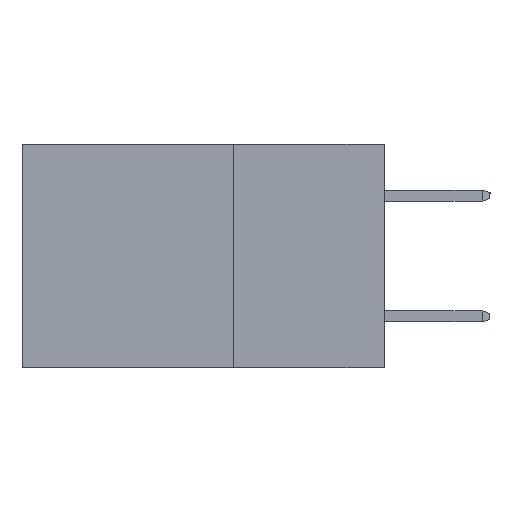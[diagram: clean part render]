
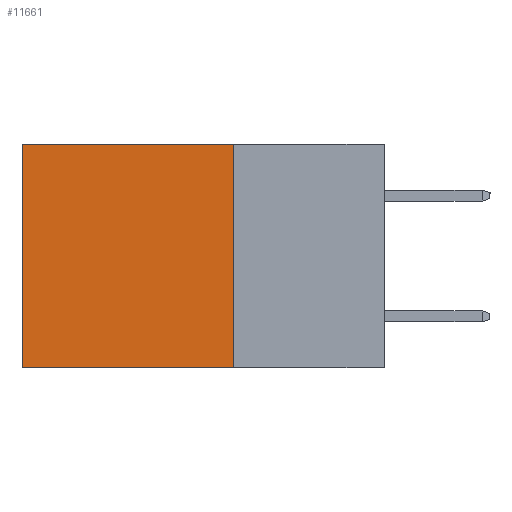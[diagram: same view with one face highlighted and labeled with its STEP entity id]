
A CAD part, left-side view. The second image highlights one B-rep face of the part: STEP entity #11661.
In plain terms, the highlighted planar face has unit normal (-1, 0, 0).
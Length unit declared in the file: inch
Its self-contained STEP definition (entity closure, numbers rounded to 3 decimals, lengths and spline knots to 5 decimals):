
#62 = LINE ( 'NONE', #4975, #13554 ) ;
#222 = EDGE_CURVE ( 'NONE', #4156, #1434, #7986, .T. ) ;
#230 = VERTEX_POINT ( 'NONE', #12919 ) ;
#1212 = CARTESIAN_POINT ( 'NONE',  ( 0.2615, 0.25, 0. ) ) ;
#1434 = VERTEX_POINT ( 'NONE', #3114 ) ;
#1591 = EDGE_CURVE ( 'NONE', #6395, #4156, #9909, .T. ) ;
#1595 = DIRECTION ( 'NONE',  ( 0., 0., -1. ) ) ;
#2038 = VECTOR ( 'NONE', #6768, 39.37008 ) ;
#2165 = PLANE ( 'NONE',  #11972 ) ;
#3040 = CARTESIAN_POINT ( 'NONE',  ( 0.2615, 0.6, -0.37 ) ) ;
#3114 = CARTESIAN_POINT ( 'NONE',  ( 0.2615, 0.6, -0.37 ) ) ;
#4156 = VERTEX_POINT ( 'NONE', #8247 ) ;
#4810 = CARTESIAN_POINT ( 'NONE',  ( 0.2615, 0.25, 0. ) ) ;
#4944 = ORIENTED_EDGE ( 'NONE', *, *, #222, .T. ) ;
#4975 = CARTESIAN_POINT ( 'NONE',  ( 0.2615, 0.25, -0.37 ) ) ;
#5056 = DIRECTION ( 'NONE',  ( 0., 1., 0. ) ) ;
#6395 = VERTEX_POINT ( 'NONE', #1212 ) ;
#6768 = DIRECTION ( 'NONE',  ( 0., 0., -1. ) ) ;
#7550 = ORIENTED_EDGE ( 'NONE', *, *, #1591, .T. ) ;
#7751 = LINE ( 'NONE', #9049, #14523 ) ;
#7986 = LINE ( 'NONE', #3040, #2038 ) ;
#8247 = CARTESIAN_POINT ( 'NONE',  ( 0.2615, 0.6, 0. ) ) ;
#9049 = CARTESIAN_POINT ( 'NONE',  ( 0.2615, 0.25, -0.37 ) ) ;
#9702 = CARTESIAN_POINT ( 'NONE',  ( 0.2615, 0.25, -0.37 ) ) ;
#9909 = LINE ( 'NONE', #4810, #14846 ) ;
#9917 = EDGE_CURVE ( 'NONE', #6395, #230, #7751, .T. ) ;
#11661 = ADVANCED_FACE ( 'NONE', ( #12126 ), #2165, .F. ) ;
#11972 = AXIS2_PLACEMENT_3D ( 'NONE', #9702, #14629, #13575 ) ;
#12126 = FACE_OUTER_BOUND ( 'NONE', #12858, .T. ) ;
#12858 = EDGE_LOOP ( 'NONE', ( #4944, #14892, #14416, #7550 ) ) ;
#12919 = CARTESIAN_POINT ( 'NONE',  ( 0.2615, 0.25, -0.37 ) ) ;
#13554 = VECTOR ( 'NONE', #5056, 39.37008 ) ;
#13575 = DIRECTION ( 'NONE',  ( 0., 0., -1. ) ) ;
#14416 = ORIENTED_EDGE ( 'NONE', *, *, #9917, .F. ) ;
#14523 = VECTOR ( 'NONE', #1595, 39.37008 ) ;
#14629 = DIRECTION ( 'NONE',  ( 1., 0., 0. ) ) ;
#14766 = DIRECTION ( 'NONE',  ( 0., 1., 0. ) ) ;
#14846 = VECTOR ( 'NONE', #14766, 39.37008 ) ;
#14848 = EDGE_CURVE ( 'NONE', #230, #1434, #62, .T. ) ;
#14892 = ORIENTED_EDGE ( 'NONE', *, *, #14848, .F. ) ;
